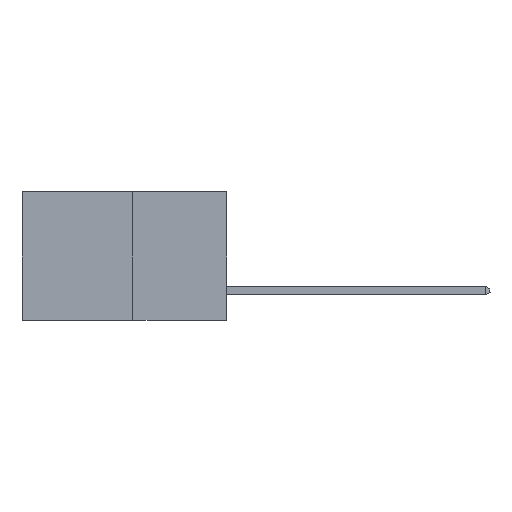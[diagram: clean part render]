
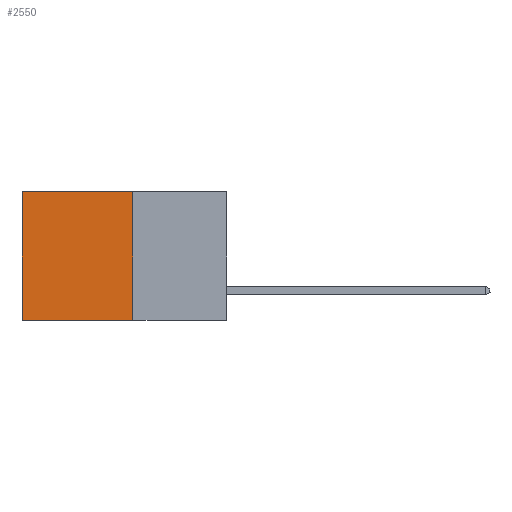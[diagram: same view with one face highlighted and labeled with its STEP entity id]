
A CAD part, left-side view. The second image highlights one B-rep face of the part: STEP entity #2550.
In plain terms, the highlighted planar face has unit normal (-1, 0, 0).
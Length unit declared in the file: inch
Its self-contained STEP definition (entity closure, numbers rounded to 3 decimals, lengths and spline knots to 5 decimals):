
#260 = ORIENTED_EDGE ( 'NONE', *, *, #19463, .F. ) ;
#1352 = ORIENTED_EDGE ( 'NONE', *, *, #4079, .T. ) ;
#1740 = VERTEX_POINT ( 'NONE', #15785 ) ;
#1978 = VECTOR ( 'NONE', #6732, 39.37008 ) ;
#2496 = LINE ( 'NONE', #5152, #1978 ) ;
#2550 = ADVANCED_FACE ( 'NONE', ( #12740 ), #18850, .F. ) ;
#3412 = CARTESIAN_POINT ( 'NONE',  ( 0.277, 0.27, -0.37 ) ) ;
#4079 = EDGE_CURVE ( 'NONE', #5571, #14390, #14218, .T. ) ;
#4561 = DIRECTION ( 'NONE',  ( 0., 1., 0. ) ) ;
#5152 = CARTESIAN_POINT ( 'NONE',  ( 0.277, 0.27, -0.37 ) ) ;
#5217 = VERTEX_POINT ( 'NONE', #3412 ) ;
#5571 = VERTEX_POINT ( 'NONE', #14239 ) ;
#5647 = LINE ( 'NONE', #9733, #13602 ) ;
#5761 = VECTOR ( 'NONE', #16544, 39.37008 ) ;
#6258 = EDGE_LOOP ( 'NONE', ( #1352, #260, #9796, #13126 ) ) ;
#6284 = VECTOR ( 'NONE', #4561, 39.37008 ) ;
#6635 = EDGE_CURVE ( 'NONE', #1740, #5217, #5647, .T. ) ;
#6732 = DIRECTION ( 'NONE',  ( 0., 1., 0. ) ) ;
#8647 = CARTESIAN_POINT ( 'NONE',  ( 0.277, 0.59, -0.37 ) ) ;
#9733 = CARTESIAN_POINT ( 'NONE',  ( 0.277, 0.27, -0.37 ) ) ;
#9796 = ORIENTED_EDGE ( 'NONE', *, *, #6635, .F. ) ;
#11781 = CARTESIAN_POINT ( 'NONE',  ( 0.277, 0.59, -0.37 ) ) ;
#12740 = FACE_OUTER_BOUND ( 'NONE', #6258, .T. ) ;
#13126 = ORIENTED_EDGE ( 'NONE', *, *, #20456, .T. ) ;
#13602 = VECTOR ( 'NONE', #14542, 39.37008 ) ;
#14073 = CARTESIAN_POINT ( 'NONE',  ( 0.277, 0.27, 0. ) ) ;
#14218 = LINE ( 'NONE', #11781, #5761 ) ;
#14239 = CARTESIAN_POINT ( 'NONE',  ( 0.277, 0.59, 0. ) ) ;
#14250 = LINE ( 'NONE', #14073, #6284 ) ;
#14390 = VERTEX_POINT ( 'NONE', #8647 ) ;
#14499 = AXIS2_PLACEMENT_3D ( 'NONE', #18976, #18621, #18702 ) ;
#14542 = DIRECTION ( 'NONE',  ( 0., 0., -1. ) ) ;
#15785 = CARTESIAN_POINT ( 'NONE',  ( 0.277, 0.27, 0. ) ) ;
#16544 = DIRECTION ( 'NONE',  ( 0., 0., -1. ) ) ;
#18621 = DIRECTION ( 'NONE',  ( 1., 0., 0. ) ) ;
#18702 = DIRECTION ( 'NONE',  ( 0., 0., -1. ) ) ;
#18850 = PLANE ( 'NONE',  #14499 ) ;
#18976 = CARTESIAN_POINT ( 'NONE',  ( 0.277, 0.27, -0.37 ) ) ;
#19463 = EDGE_CURVE ( 'NONE', #5217, #14390, #2496, .T. ) ;
#20456 = EDGE_CURVE ( 'NONE', #1740, #5571, #14250, .T. ) ;
